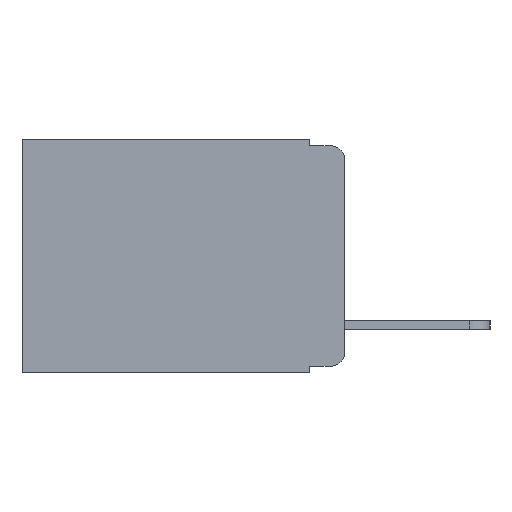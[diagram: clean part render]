
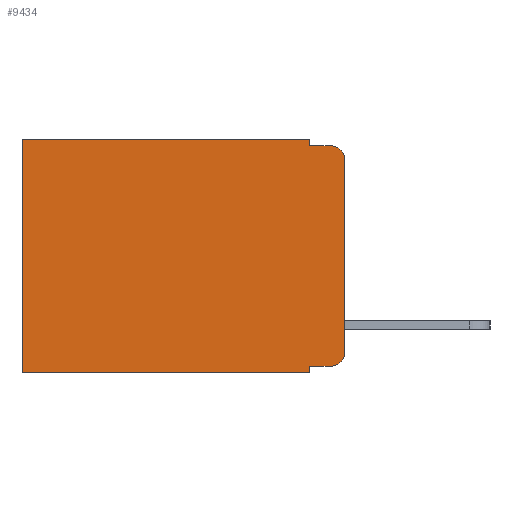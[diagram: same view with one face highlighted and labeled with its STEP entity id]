
A CAD part, left-side view. The second image highlights one B-rep face of the part: STEP entity #9434.
In plain terms, the highlighted planar face has unit normal (-1, 0, 0).
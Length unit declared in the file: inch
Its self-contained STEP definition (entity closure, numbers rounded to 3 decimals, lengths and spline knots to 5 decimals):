
#67 = VERTEX_POINT ( 'NONE', #11601 ) ;
#81 = CARTESIAN_POINT ( 'NONE',  ( 0.298, 0., 0. ) ) ;
#181 = LINE ( 'NONE', #3127, #6246 ) ;
#256 = LINE ( 'NONE', #7135, #12036 ) ;
#516 = EDGE_CURVE ( 'NONE', #13615, #1539, #256, .T. ) ;
#943 = AXIS2_PLACEMENT_3D ( 'NONE', #9238, #1060, #9295 ) ;
#1060 = DIRECTION ( 'NONE',  ( -1., 0., 0. ) ) ;
#1535 = LINE ( 'NONE', #4181, #10369 ) ;
#1539 = VERTEX_POINT ( 'NONE', #14231 ) ;
#1684 = CARTESIAN_POINT ( 'NONE',  ( 0.298, 0.02, -0.333 ) ) ;
#1924 = ORIENTED_EDGE ( 'NONE', *, *, #8416, .T. ) ;
#1983 = LINE ( 'NONE', #9504, #7178 ) ;
#2021 = ORIENTED_EDGE ( 'NONE', *, *, #9151, .F. ) ;
#2450 = DIRECTION ( 'NONE',  ( 0., 0., -1. ) ) ;
#2502 = VERTEX_POINT ( 'NONE', #5617 ) ;
#2930 = CARTESIAN_POINT ( 'NONE',  ( 0.298, 0., -0.03 ) ) ;
#2968 = VERTEX_POINT ( 'NONE', #6603 ) ;
#3127 = CARTESIAN_POINT ( 'NONE',  ( 0.298, 0.051, 0. ) ) ;
#3288 = ORIENTED_EDGE ( 'NONE', *, *, #516, .F. ) ;
#3640 = CARTESIAN_POINT ( 'NONE',  ( 0.298, 0., 0. ) ) ;
#3974 = CARTESIAN_POINT ( 'NONE',  ( 0.298, 0.473, 0. ) ) ;
#4181 = CARTESIAN_POINT ( 'NONE',  ( 0.298, 0.051, -0.01 ) ) ;
#4333 = ORIENTED_EDGE ( 'NONE', *, *, #10196, .T. ) ;
#4472 = CARTESIAN_POINT ( 'NONE',  ( 0.298, 0.473, -0.343 ) ) ;
#4635 = DIRECTION ( 'NONE',  ( 0., 1., 0. ) ) ;
#4866 = EDGE_CURVE ( 'NONE', #6963, #2502, #7753, .T. ) ;
#4962 = EDGE_CURVE ( 'NONE', #13389, #67, #6275, .T. ) ;
#5252 = CARTESIAN_POINT ( 'NONE',  ( 0.298, 0., -0.343 ) ) ;
#5617 = CARTESIAN_POINT ( 'NONE',  ( 0.298, 0.02, -0.01 ) ) ;
#5702 = VECTOR ( 'NONE', #8502, 39.37008 ) ;
#5907 = DIRECTION ( 'NONE',  ( 0., 0., -1. ) ) ;
#6169 = DIRECTION ( 'NONE',  ( 0., 0., -1. ) ) ;
#6205 = CARTESIAN_POINT ( 'NONE',  ( 0.298, 0.051, -0.01 ) ) ;
#6213 = EDGE_CURVE ( 'NONE', #13615, #11856, #1983, .T. ) ;
#6246 = VECTOR ( 'NONE', #12469, 39.37008 ) ;
#6275 = LINE ( 'NONE', #81, #9233 ) ;
#6603 = CARTESIAN_POINT ( 'NONE',  ( 0.298, 0., -0.313 ) ) ;
#6963 = VERTEX_POINT ( 'NONE', #2930 ) ;
#6977 = AXIS2_PLACEMENT_3D ( 'NONE', #10767, #7252, #2450 ) ;
#7070 = ORIENTED_EDGE ( 'NONE', *, *, #4866, .T. ) ;
#7135 = CARTESIAN_POINT ( 'NONE',  ( 0.298, 0.051, 0. ) ) ;
#7178 = VECTOR ( 'NONE', #7294, 39.37008 ) ;
#7191 = ORIENTED_EDGE ( 'NONE', *, *, #8510, .F. ) ;
#7252 = DIRECTION ( 'NONE',  ( 1., 0., 0. ) ) ;
#7294 = DIRECTION ( 'NONE',  ( 0., -1., 0. ) ) ;
#7442 = ORIENTED_EDGE ( 'NONE', *, *, #13775, .F. ) ;
#7514 = CIRCLE ( 'NONE', #9538, 0.02 ) ;
#7524 = EDGE_CURVE ( 'NONE', #6963, #2968, #9078, .T. ) ;
#7555 = VERTEX_POINT ( 'NONE', #4472 ) ;
#7556 = DIRECTION ( 'NONE',  ( 0., 0., -1. ) ) ;
#7573 = LINE ( 'NONE', #3974, #5702 ) ;
#7753 = CIRCLE ( 'NONE', #943, 0.02 ) ;
#8416 = EDGE_CURVE ( 'NONE', #67, #7555, #7573, .T. ) ;
#8502 = DIRECTION ( 'NONE',  ( 0., 0., -1. ) ) ;
#8510 = EDGE_CURVE ( 'NONE', #1539, #7555, #11274, .T. ) ;
#8522 = DIRECTION ( 'NONE',  ( -1., 0., 0. ) ) ;
#8633 = FACE_OUTER_BOUND ( 'NONE', #9209, .T. ) ;
#9078 = LINE ( 'NONE', #3640, #13135 ) ;
#9151 = EDGE_CURVE ( 'NONE', #13389, #10241, #181, .T. ) ;
#9209 = EDGE_LOOP ( 'NONE', ( #11992, #7070, #7442, #2021, #12324, #1924, #7191, #3288, #14782, #4333 ) ) ;
#9233 = VECTOR ( 'NONE', #4635, 39.37008 ) ;
#9238 = CARTESIAN_POINT ( 'NONE',  ( 0.298, 0.02, -0.03 ) ) ;
#9295 = DIRECTION ( 'NONE',  ( 0., 0., -1. ) ) ;
#9322 = CARTESIAN_POINT ( 'NONE',  ( 0.298, 0.051, 0. ) ) ;
#9434 = ADVANCED_FACE ( 'NONE', ( #8633 ), #14201, .F. ) ;
#9504 = CARTESIAN_POINT ( 'NONE',  ( 0.298, 0.051, -0.333 ) ) ;
#9538 = AXIS2_PLACEMENT_3D ( 'NONE', #10973, #8522, #7556 ) ;
#9839 = CARTESIAN_POINT ( 'NONE',  ( 0.298, 0.051, -0.333 ) ) ;
#10196 = EDGE_CURVE ( 'NONE', #11856, #2968, #7514, .T. ) ;
#10241 = VERTEX_POINT ( 'NONE', #6205 ) ;
#10369 = VECTOR ( 'NONE', #12438, 39.37008 ) ;
#10767 = CARTESIAN_POINT ( 'NONE',  ( 0.298, 0., 0. ) ) ;
#10973 = CARTESIAN_POINT ( 'NONE',  ( 0.298, 0.02, -0.313 ) ) ;
#11274 = LINE ( 'NONE', #5252, #13278 ) ;
#11601 = CARTESIAN_POINT ( 'NONE',  ( 0.298, 0.473, 0. ) ) ;
#11856 = VERTEX_POINT ( 'NONE', #1684 ) ;
#11992 = ORIENTED_EDGE ( 'NONE', *, *, #7524, .F. ) ;
#12036 = VECTOR ( 'NONE', #6169, 39.37008 ) ;
#12324 = ORIENTED_EDGE ( 'NONE', *, *, #4962, .T. ) ;
#12438 = DIRECTION ( 'NONE',  ( 0., -1., 0. ) ) ;
#12469 = DIRECTION ( 'NONE',  ( 0., 0., -1. ) ) ;
#12474 = DIRECTION ( 'NONE',  ( 0., 1., 0. ) ) ;
#13135 = VECTOR ( 'NONE', #5907, 39.37008 ) ;
#13278 = VECTOR ( 'NONE', #12474, 39.37008 ) ;
#13389 = VERTEX_POINT ( 'NONE', #9322 ) ;
#13615 = VERTEX_POINT ( 'NONE', #9839 ) ;
#13775 = EDGE_CURVE ( 'NONE', #10241, #2502, #1535, .T. ) ;
#14201 = PLANE ( 'NONE',  #6977 ) ;
#14231 = CARTESIAN_POINT ( 'NONE',  ( 0.298, 0.051, -0.343 ) ) ;
#14782 = ORIENTED_EDGE ( 'NONE', *, *, #6213, .T. ) ;
